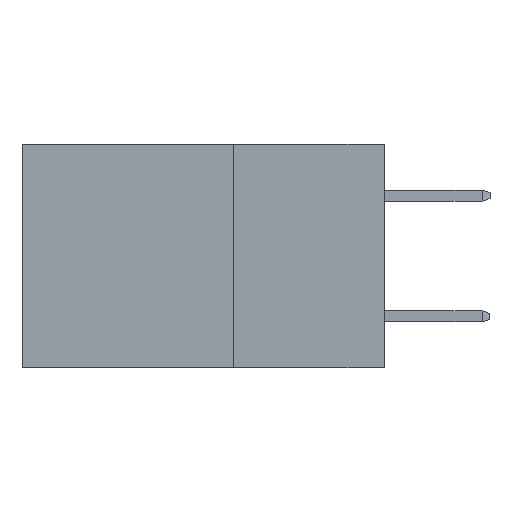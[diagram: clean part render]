
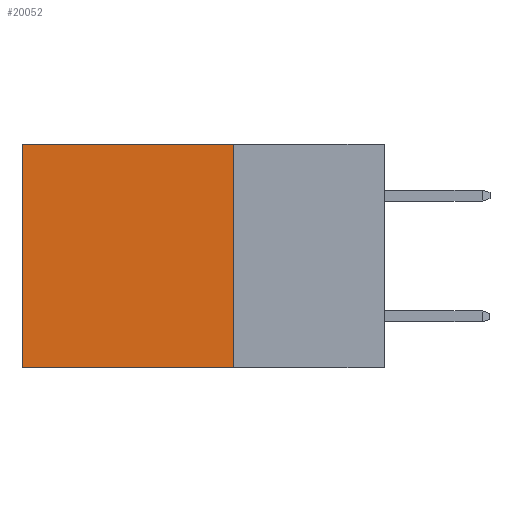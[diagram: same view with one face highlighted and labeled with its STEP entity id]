
A CAD part, left-side view. The second image highlights one B-rep face of the part: STEP entity #20052.
In plain terms, the highlighted planar face has unit normal (-1, 0, 0).
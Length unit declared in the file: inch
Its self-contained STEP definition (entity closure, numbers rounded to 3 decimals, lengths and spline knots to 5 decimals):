
#715 = ORIENTED_EDGE ( 'NONE', *, *, #22172, .F. ) ;
#736 = DIRECTION ( 'NONE',  ( 0., 1., 0. ) ) ;
#1498 = AXIS2_PLACEMENT_3D ( 'NONE', #16587, #4765, #18574 ) ;
#1647 = VERTEX_POINT ( 'NONE', #16012 ) ;
#3514 = CARTESIAN_POINT ( 'NONE',  ( 0.298, 0.25, -0.37 ) ) ;
#4765 = DIRECTION ( 'NONE',  ( 1., 0., 0. ) ) ;
#5123 = EDGE_CURVE ( 'NONE', #15906, #14507, #9761, .T. ) ;
#5599 = ORIENTED_EDGE ( 'NONE', *, *, #8274, .T. ) ;
#5788 = EDGE_CURVE ( 'NONE', #1647, #14507, #10036, .T. ) ;
#6062 = LINE ( 'NONE', #24276, #10717 ) ;
#8274 = EDGE_CURVE ( 'NONE', #19964, #1647, #6062, .T. ) ;
#9414 = VECTOR ( 'NONE', #10601, 39.37008 ) ;
#9761 = LINE ( 'NONE', #20065, #14362 ) ;
#10036 = LINE ( 'NONE', #20397, #9414 ) ;
#10601 = DIRECTION ( 'NONE',  ( 0., 0., -1. ) ) ;
#10717 = VECTOR ( 'NONE', #736, 39.37008 ) ;
#14090 = CARTESIAN_POINT ( 'NONE',  ( 0.298, 0.25, 0. ) ) ;
#14362 = VECTOR ( 'NONE', #20154, 39.37008 ) ;
#14507 = VERTEX_POINT ( 'NONE', #24650 ) ;
#15906 = VERTEX_POINT ( 'NONE', #3514 ) ;
#16012 = CARTESIAN_POINT ( 'NONE',  ( 0.298, 0.6, 0. ) ) ;
#16587 = CARTESIAN_POINT ( 'NONE',  ( 0.298, 0.25, 0. ) ) ;
#18428 = EDGE_LOOP ( 'NONE', ( #24181, #22951, #715, #5599 ) ) ;
#18574 = DIRECTION ( 'NONE',  ( 0., 0., -1. ) ) ;
#19964 = VERTEX_POINT ( 'NONE', #22157 ) ;
#20052 = ADVANCED_FACE ( 'NONE', ( #21805 ), #24347, .F. ) ;
#20065 = CARTESIAN_POINT ( 'NONE',  ( 0.298, 0.25, -0.37 ) ) ;
#20154 = DIRECTION ( 'NONE',  ( 0., 1., 0. ) ) ;
#20397 = CARTESIAN_POINT ( 'NONE',  ( 0.298, 0.6, 0. ) ) ;
#21805 = FACE_OUTER_BOUND ( 'NONE', #18428, .T. ) ;
#22157 = CARTESIAN_POINT ( 'NONE',  ( 0.298, 0.25, 0. ) ) ;
#22172 = EDGE_CURVE ( 'NONE', #19964, #15906, #24725, .T. ) ;
#22951 = ORIENTED_EDGE ( 'NONE', *, *, #5123, .F. ) ;
#23916 = DIRECTION ( 'NONE',  ( 0., 0., -1. ) ) ;
#24106 = VECTOR ( 'NONE', #23916, 39.37008 ) ;
#24181 = ORIENTED_EDGE ( 'NONE', *, *, #5788, .T. ) ;
#24276 = CARTESIAN_POINT ( 'NONE',  ( 0.298, 0.25, 0. ) ) ;
#24347 = PLANE ( 'NONE',  #1498 ) ;
#24650 = CARTESIAN_POINT ( 'NONE',  ( 0.298, 0.6, -0.37 ) ) ;
#24725 = LINE ( 'NONE', #14090, #24106 ) ;
